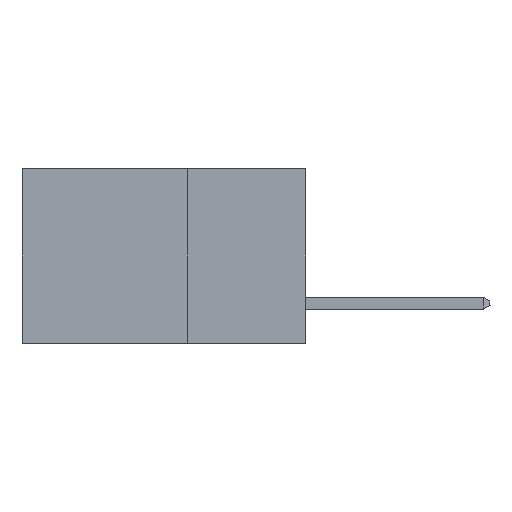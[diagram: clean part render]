
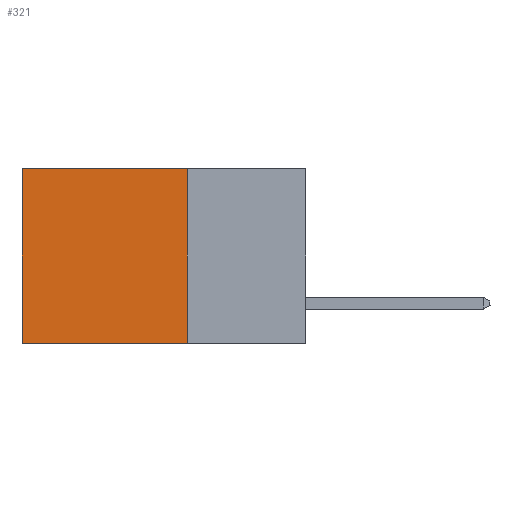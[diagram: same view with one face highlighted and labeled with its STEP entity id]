
A CAD part, left-side view. The second image highlights one B-rep face of the part: STEP entity #321.
In plain terms, the highlighted planar face has unit normal (-1, 0, 0).
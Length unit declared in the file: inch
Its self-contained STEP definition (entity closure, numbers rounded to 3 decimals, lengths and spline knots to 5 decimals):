
#321 = ADVANCED_FACE ( 'NONE', ( #871 ), #20704, .F. ) ;
#871 = FACE_OUTER_BOUND ( 'NONE', #14054, .T. ) ;
#1117 = DIRECTION ( 'NONE',  ( 1., 0., 0. ) ) ;
#1675 = CARTESIAN_POINT ( 'NONE',  ( 0.298, 0.25, 0. ) ) ;
#2476 = CARTESIAN_POINT ( 'NONE',  ( 0.298, 0.25, 0. ) ) ;
#3133 = LINE ( 'NONE', #24273, #19064 ) ;
#4986 = VERTEX_POINT ( 'NONE', #18439 ) ;
#9283 = VERTEX_POINT ( 'NONE', #15215 ) ;
#9867 = VECTOR ( 'NONE', #21964, 39.37008 ) ;
#10581 = VERTEX_POINT ( 'NONE', #10886 ) ;
#10886 = CARTESIAN_POINT ( 'NONE',  ( 0.298, 0.6, 0. ) ) ;
#11766 = ORIENTED_EDGE ( 'NONE', *, *, #12219, .T. ) ;
#12140 = DIRECTION ( 'NONE',  ( 0., 1., 0. ) ) ;
#12219 = EDGE_CURVE ( 'NONE', #10581, #9283, #21178, .T. ) ;
#12561 = CARTESIAN_POINT ( 'NONE',  ( 0.298, 0.25, 0. ) ) ;
#14051 = DIRECTION ( 'NONE',  ( 0., 1., 0. ) ) ;
#14054 = EDGE_LOOP ( 'NONE', ( #11766, #20157, #25262, #25570 ) ) ;
#15215 = CARTESIAN_POINT ( 'NONE',  ( 0.298, 0.6, -0.37 ) ) ;
#15246 = VERTEX_POINT ( 'NONE', #2476 ) ;
#15964 = DIRECTION ( 'NONE',  ( 0., 0., -1. ) ) ;
#16370 = EDGE_CURVE ( 'NONE', #15246, #10581, #16630, .T. ) ;
#16630 = LINE ( 'NONE', #1675, #20928 ) ;
#17175 = EDGE_CURVE ( 'NONE', #15246, #4986, #23151, .T. ) ;
#18028 = DIRECTION ( 'NONE',  ( 0., 0., -1. ) ) ;
#18439 = CARTESIAN_POINT ( 'NONE',  ( 0.298, 0.25, -0.37 ) ) ;
#19064 = VECTOR ( 'NONE', #14051, 39.37008 ) ;
#20143 = VECTOR ( 'NONE', #18028, 39.37008 ) ;
#20157 = ORIENTED_EDGE ( 'NONE', *, *, #24549, .F. ) ;
#20158 = CARTESIAN_POINT ( 'NONE',  ( 0.298, 0.25, 0. ) ) ;
#20704 = PLANE ( 'NONE',  #23450 ) ;
#20928 = VECTOR ( 'NONE', #12140, 39.37008 ) ;
#21178 = LINE ( 'NONE', #22375, #9867 ) ;
#21964 = DIRECTION ( 'NONE',  ( 0., 0., -1. ) ) ;
#22375 = CARTESIAN_POINT ( 'NONE',  ( 0.298, 0.6, 0. ) ) ;
#23151 = LINE ( 'NONE', #20158, #20143 ) ;
#23450 = AXIS2_PLACEMENT_3D ( 'NONE', #12561, #1117, #15964 ) ;
#24273 = CARTESIAN_POINT ( 'NONE',  ( 0.298, 0.25, -0.37 ) ) ;
#24549 = EDGE_CURVE ( 'NONE', #4986, #9283, #3133, .T. ) ;
#25262 = ORIENTED_EDGE ( 'NONE', *, *, #17175, .F. ) ;
#25570 = ORIENTED_EDGE ( 'NONE', *, *, #16370, .T. ) ;
